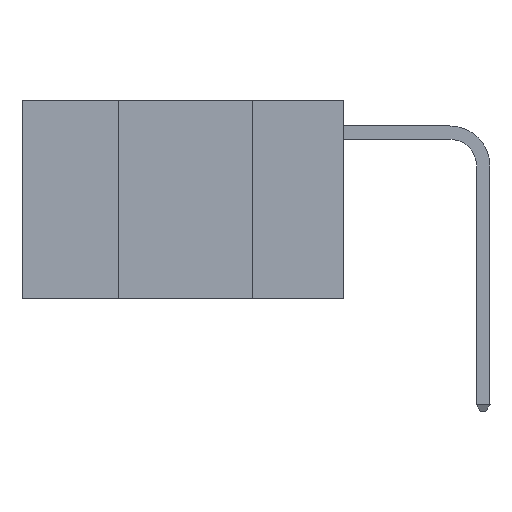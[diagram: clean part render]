
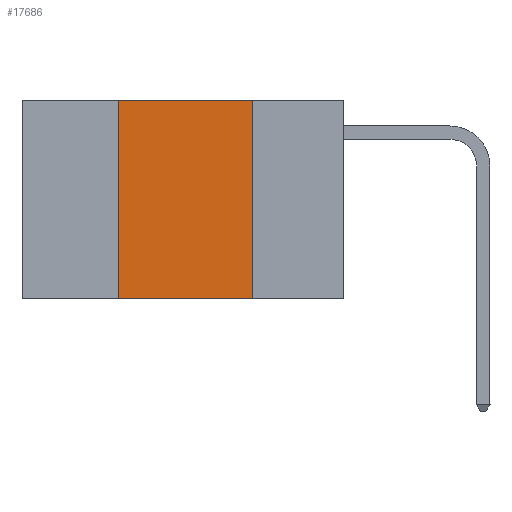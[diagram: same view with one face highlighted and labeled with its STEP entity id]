
A CAD part, left-side view. The second image highlights one B-rep face of the part: STEP entity #17686.
In plain terms, the highlighted planar face has unit normal (-1, 0, 0).
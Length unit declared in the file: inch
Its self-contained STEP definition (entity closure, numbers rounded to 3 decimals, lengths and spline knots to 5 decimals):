
#1193 = VERTEX_POINT ( 'NONE', #18202 ) ;
#4057 = PLANE ( 'NONE',  #20641 ) ;
#4683 = DIRECTION ( 'NONE',  ( 0., -1., 0. ) ) ;
#5054 = VECTOR ( 'NONE', #21052, 39.37008 ) ;
#6036 = VERTEX_POINT ( 'NONE', #22319 ) ;
#7152 = LINE ( 'NONE', #24929, #11803 ) ;
#8433 = CARTESIAN_POINT ( 'NONE',  ( 0., 0.42, 0. ) ) ;
#8488 = VECTOR ( 'NONE', #4683, 39.37008 ) ;
#10090 = DIRECTION ( 'NONE',  ( 0., 0., -1. ) ) ;
#10392 = DIRECTION ( 'NONE',  ( 0., 0., 1. ) ) ;
#10518 = CARTESIAN_POINT ( 'NONE',  ( 0., 0.17, 0. ) ) ;
#11803 = VECTOR ( 'NONE', #14925, 39.37008 ) ;
#12626 = CARTESIAN_POINT ( 'NONE',  ( 0., 0.6, -0.37 ) ) ;
#12780 = VECTOR ( 'NONE', #10392, 39.37008 ) ;
#13394 = LINE ( 'NONE', #8433, #12780 ) ;
#14008 = CARTESIAN_POINT ( 'NONE',  ( 0., 0.6, 0. ) ) ;
#14925 = DIRECTION ( 'NONE',  ( 0., -1., 0. ) ) ;
#15022 = LINE ( 'NONE', #12626, #8488 ) ;
#15246 = VERTEX_POINT ( 'NONE', #10518 ) ;
#15301 = EDGE_CURVE ( 'NONE', #15607, #6036, #15022, .T. ) ;
#15607 = VERTEX_POINT ( 'NONE', #25573 ) ;
#15673 = LINE ( 'NONE', #19030, #5054 ) ;
#16642 = EDGE_CURVE ( 'NONE', #15607, #1193, #13394, .T. ) ;
#16699 = ORIENTED_EDGE ( 'NONE', *, *, #20683, .F. ) ;
#17186 = ORIENTED_EDGE ( 'NONE', *, *, #17347, .F. ) ;
#17347 = EDGE_CURVE ( 'NONE', #1193, #15246, #7152, .T. ) ;
#17686 = ADVANCED_FACE ( 'NONE', ( #24353 ), #4057, .F. ) ;
#18202 = CARTESIAN_POINT ( 'NONE',  ( 0., 0.42, 0. ) ) ;
#19030 = CARTESIAN_POINT ( 'NONE',  ( 0., 0.17, 0. ) ) ;
#20190 = ORIENTED_EDGE ( 'NONE', *, *, #16642, .F. ) ;
#20641 = AXIS2_PLACEMENT_3D ( 'NONE', #14008, #22107, #10090 ) ;
#20683 = EDGE_CURVE ( 'NONE', #15246, #6036, #15673, .T. ) ;
#21052 = DIRECTION ( 'NONE',  ( 0., 0., -1. ) ) ;
#21869 = ORIENTED_EDGE ( 'NONE', *, *, #15301, .T. ) ;
#22107 = DIRECTION ( 'NONE',  ( 1., 0., 0. ) ) ;
#22148 = EDGE_LOOP ( 'NONE', ( #16699, #17186, #20190, #21869 ) ) ;
#22319 = CARTESIAN_POINT ( 'NONE',  ( 0., 0.17, -0.37 ) ) ;
#24353 = FACE_OUTER_BOUND ( 'NONE', #22148, .T. ) ;
#24929 = CARTESIAN_POINT ( 'NONE',  ( 0., 0.6, 0. ) ) ;
#25573 = CARTESIAN_POINT ( 'NONE',  ( 0., 0.42, -0.37 ) ) ;
